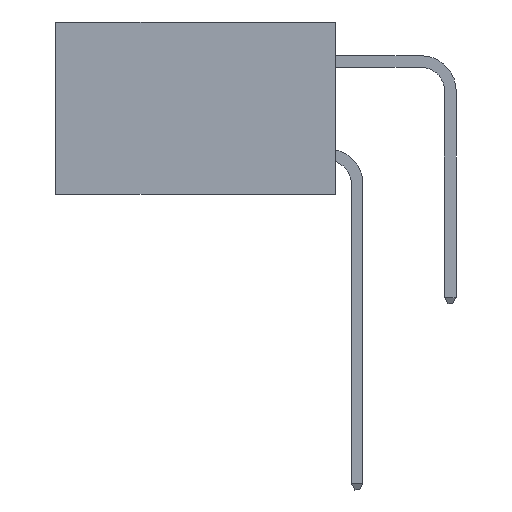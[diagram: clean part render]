
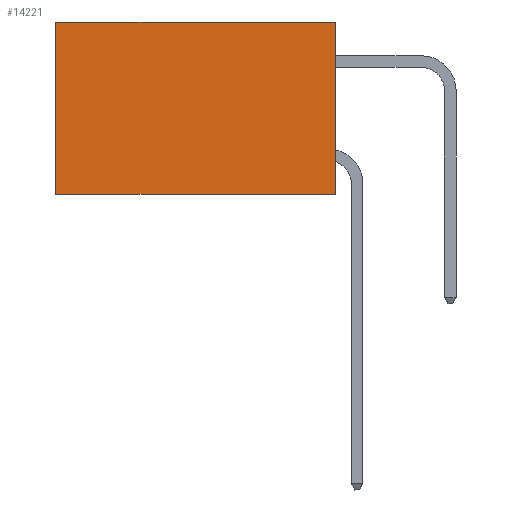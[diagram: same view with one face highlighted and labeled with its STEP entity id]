
A CAD part, left-side view. The second image highlights one B-rep face of the part: STEP entity #14221.
In plain terms, the highlighted planar face has unit normal (-1, 0, 0).
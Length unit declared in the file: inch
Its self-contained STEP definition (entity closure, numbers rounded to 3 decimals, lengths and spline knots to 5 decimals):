
#130 = CARTESIAN_POINT ( 'NONE',  ( 0.2875, 0., -0.37 ) ) ;
#573 = VECTOR ( 'NONE', #3001, 39.37008 ) ;
#877 = LINE ( 'NONE', #30611, #27244 ) ;
#1358 = DIRECTION ( 'NONE',  ( 1., 0., 0. ) ) ;
#1638 = VECTOR ( 'NONE', #11694, 39.37008 ) ;
#2827 = EDGE_CURVE ( 'NONE', #6647, #17228, #16899, .T. ) ;
#3001 = DIRECTION ( 'NONE',  ( 0., 1., 0. ) ) ;
#3427 = CARTESIAN_POINT ( 'NONE',  ( 0.2875, 0., 0. ) ) ;
#4495 = ORIENTED_EDGE ( 'NONE', *, *, #27713, .T. ) ;
#6647 = VERTEX_POINT ( 'NONE', #12341 ) ;
#7619 = LINE ( 'NONE', #12029, #1638 ) ;
#10214 = VERTEX_POINT ( 'NONE', #3427 ) ;
#10503 = VERTEX_POINT ( 'NONE', #14868 ) ;
#11694 = DIRECTION ( 'NONE',  ( 0., 0., -1. ) ) ;
#11956 = CARTESIAN_POINT ( 'NONE',  ( 0.2875, 0., 0. ) ) ;
#12029 = CARTESIAN_POINT ( 'NONE',  ( 0.2875, 0., 0. ) ) ;
#12341 = CARTESIAN_POINT ( 'NONE',  ( 0.2875, 0., -0.37 ) ) ;
#12918 = ORIENTED_EDGE ( 'NONE', *, *, #15238, .F. ) ;
#13020 = DIRECTION ( 'NONE',  ( 0., 0., -1. ) ) ;
#14221 = ADVANCED_FACE ( 'NONE', ( #22570 ), #27255, .F. ) ;
#14868 = CARTESIAN_POINT ( 'NONE',  ( 0.2875, 0.6, 0. ) ) ;
#14973 = ORIENTED_EDGE ( 'NONE', *, *, #2827, .F. ) ;
#15238 = EDGE_CURVE ( 'NONE', #10214, #6647, #7619, .T. ) ;
#15326 = ORIENTED_EDGE ( 'NONE', *, *, #18476, .T. ) ;
#16899 = LINE ( 'NONE', #130, #573 ) ;
#17042 = DIRECTION ( 'NONE',  ( 0., 1., 0. ) ) ;
#17228 = VERTEX_POINT ( 'NONE', #22809 ) ;
#18476 = EDGE_CURVE ( 'NONE', #10214, #10503, #20929, .T. ) ;
#19205 = DIRECTION ( 'NONE',  ( 0., 0., -1. ) ) ;
#20929 = LINE ( 'NONE', #29812, #32134 ) ;
#22570 = FACE_OUTER_BOUND ( 'NONE', #29731, .T. ) ;
#22809 = CARTESIAN_POINT ( 'NONE',  ( 0.2875, 0.6, -0.37 ) ) ;
#26887 = AXIS2_PLACEMENT_3D ( 'NONE', #11956, #1358, #19205 ) ;
#27244 = VECTOR ( 'NONE', #13020, 39.37008 ) ;
#27255 = PLANE ( 'NONE',  #26887 ) ;
#27713 = EDGE_CURVE ( 'NONE', #10503, #17228, #877, .T. ) ;
#29731 = EDGE_LOOP ( 'NONE', ( #4495, #14973, #12918, #15326 ) ) ;
#29812 = CARTESIAN_POINT ( 'NONE',  ( 0.2875, 0., 0. ) ) ;
#30611 = CARTESIAN_POINT ( 'NONE',  ( 0.2875, 0.6, 0. ) ) ;
#32134 = VECTOR ( 'NONE', #17042, 39.37008 ) ;
